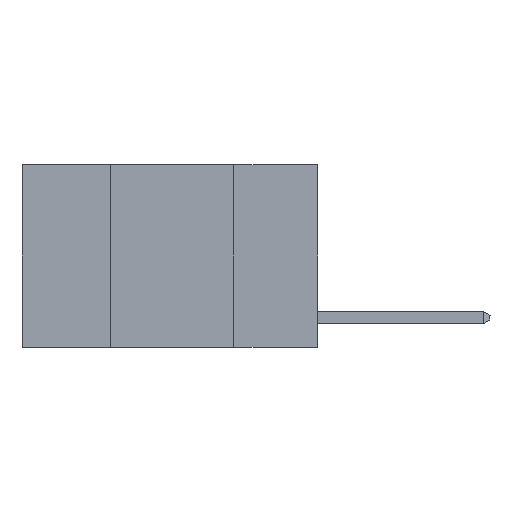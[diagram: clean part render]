
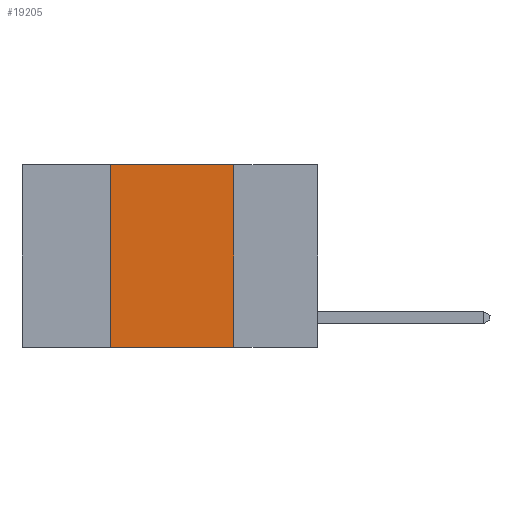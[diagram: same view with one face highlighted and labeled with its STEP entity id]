
A CAD part, left-side view. The second image highlights one B-rep face of the part: STEP entity #19205.
In plain terms, the highlighted planar face has unit normal (-1, 0, 0).
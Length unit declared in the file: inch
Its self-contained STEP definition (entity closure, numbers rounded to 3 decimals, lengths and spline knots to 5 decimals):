
#69 = CARTESIAN_POINT ( 'NONE',  ( 0., 0.6, -0.37 ) ) ;
#2402 = DIRECTION ( 'NONE',  ( 0., 0., -1. ) ) ;
#2448 = CARTESIAN_POINT ( 'NONE',  ( 0., 0.6, 0. ) ) ;
#3898 = VECTOR ( 'NONE', #26223, 39.37008 ) ;
#4977 = CARTESIAN_POINT ( 'NONE',  ( 0., 0.42, 0. ) ) ;
#5798 = CARTESIAN_POINT ( 'NONE',  ( 0., 0.42, 0. ) ) ;
#7917 = CARTESIAN_POINT ( 'NONE',  ( 0., 0.17, -0.37 ) ) ;
#9727 = LINE ( 'NONE', #23282, #22585 ) ;
#11283 = VECTOR ( 'NONE', #28251, 39.37008 ) ;
#11486 = CARTESIAN_POINT ( 'NONE',  ( 0., 0.17, 0. ) ) ;
#14397 = LINE ( 'NONE', #69, #11283 ) ;
#17663 = EDGE_LOOP ( 'NONE', ( #19131, #20745, #27752, #21180 ) ) ;
#17725 = CARTESIAN_POINT ( 'NONE',  ( 0., 0.6, 0. ) ) ;
#17974 = EDGE_CURVE ( 'NONE', #23774, #26052, #9727, .T. ) ;
#18922 = PLANE ( 'NONE',  #25119 ) ;
#19131 = ORIENTED_EDGE ( 'NONE', *, *, #17974, .F. ) ;
#19205 = ADVANCED_FACE ( 'NONE', ( #27739 ), #18922, .F. ) ;
#20335 = EDGE_CURVE ( 'NONE', #27653, #23774, #22883, .T. ) ;
#20745 = ORIENTED_EDGE ( 'NONE', *, *, #20335, .F. ) ;
#21180 = ORIENTED_EDGE ( 'NONE', *, *, #26838, .T. ) ;
#21814 = LINE ( 'NONE', #5798, #3898 ) ;
#22585 = VECTOR ( 'NONE', #2402, 39.37008 ) ;
#22883 = LINE ( 'NONE', #17725, #23215 ) ;
#23032 = DIRECTION ( 'NONE',  ( 1., 0., 0. ) ) ;
#23215 = VECTOR ( 'NONE', #26985, 39.37008 ) ;
#23282 = CARTESIAN_POINT ( 'NONE',  ( 0., 0.17, 0. ) ) ;
#23774 = VERTEX_POINT ( 'NONE', #11486 ) ;
#25119 = AXIS2_PLACEMENT_3D ( 'NONE', #2448, #23032, #27588 ) ;
#25814 = VERTEX_POINT ( 'NONE', #27716 ) ;
#26052 = VERTEX_POINT ( 'NONE', #7917 ) ;
#26223 = DIRECTION ( 'NONE',  ( 0., 0., 1. ) ) ;
#26838 = EDGE_CURVE ( 'NONE', #25814, #26052, #14397, .T. ) ;
#26985 = DIRECTION ( 'NONE',  ( 0., -1., 0. ) ) ;
#27445 = EDGE_CURVE ( 'NONE', #25814, #27653, #21814, .T. ) ;
#27588 = DIRECTION ( 'NONE',  ( 0., 0., -1. ) ) ;
#27653 = VERTEX_POINT ( 'NONE', #4977 ) ;
#27716 = CARTESIAN_POINT ( 'NONE',  ( 0., 0.42, -0.37 ) ) ;
#27739 = FACE_OUTER_BOUND ( 'NONE', #17663, .T. ) ;
#27752 = ORIENTED_EDGE ( 'NONE', *, *, #27445, .F. ) ;
#28251 = DIRECTION ( 'NONE',  ( 0., -1., 0. ) ) ;
